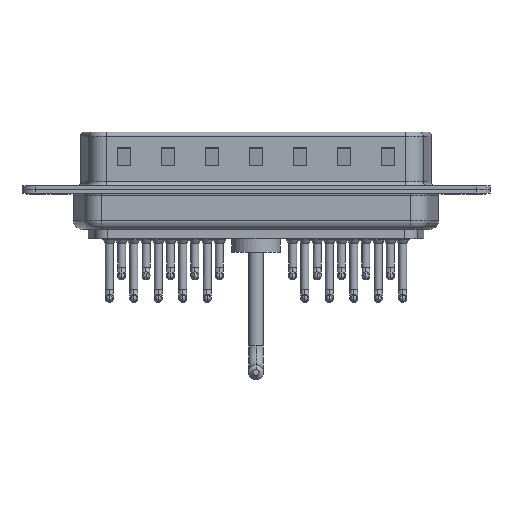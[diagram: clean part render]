
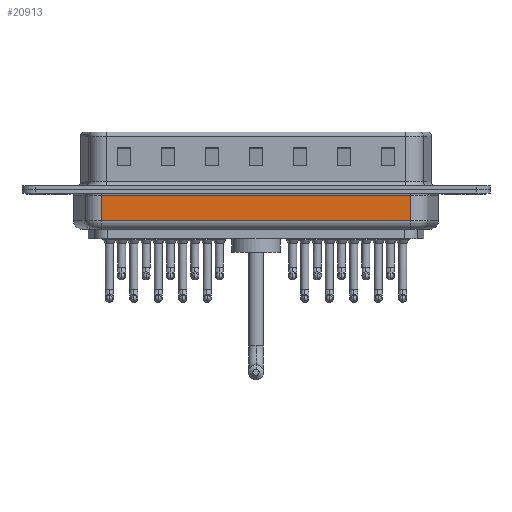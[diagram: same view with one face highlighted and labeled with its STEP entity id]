
A CAD part, front view. The second image highlights one B-rep face of the part: STEP entity #20913.
In plain terms, the highlighted planar face has unit normal (0, -1, 0).
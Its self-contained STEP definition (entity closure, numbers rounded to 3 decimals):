
#125 = CARTESIAN_POINT ( 'NONE',  ( 6.006, -5.35, -0.65 ) ) ;
#293 = ORIENTED_EDGE ( 'NONE', *, *, #11202, .T. ) ;
#4726 = CARTESIAN_POINT ( 'NONE',  ( 6.006, -5.35, -0.65 ) ) ;
#4767 = VECTOR ( 'NONE', #20008, 1000. ) ;
#5064 = FACE_OUTER_BOUND ( 'NONE', #13318, .T. ) ;
#5368 = DIRECTION ( 'NONE',  ( -1., 0., 0. ) ) ;
#5595 = LINE ( 'NONE', #125, #11075 ) ;
#6647 = ORIENTED_EDGE ( 'NONE', *, *, #16174, .T. ) ;
#6909 = VERTEX_POINT ( 'NONE', #4726 ) ;
#7134 = DIRECTION ( 'NONE',  ( 0., 1., 0. ) ) ;
#7353 = LINE ( 'NONE', #11246, #23044 ) ;
#8063 = CARTESIAN_POINT ( 'NONE',  ( 6.006, -5.35, -4.5 ) ) ;
#9010 = CARTESIAN_POINT ( 'NONE',  ( 41.044, -5.35, -3.5 ) ) ;
#9909 = EDGE_CURVE ( 'NONE', #18828, #12997, #12587, .T. ) ;
#10385 = LINE ( 'NONE', #8063, #19255 ) ;
#11061 = CARTESIAN_POINT ( 'NONE',  ( 41.044, -5.35, -0.65 ) ) ;
#11075 = VECTOR ( 'NONE', #5368, 1000. ) ;
#11202 = EDGE_CURVE ( 'NONE', #16367, #6909, #5595, .T. ) ;
#11246 = CARTESIAN_POINT ( 'NONE',  ( 41.044, -5.35, -4.5 ) ) ;
#12587 = LINE ( 'NONE', #21594, #4767 ) ;
#12738 = DIRECTION ( 'NONE',  ( 0., 0., 1. ) ) ;
#12997 = VERTEX_POINT ( 'NONE', #9010 ) ;
#13318 = EDGE_LOOP ( 'NONE', ( #19593, #15335, #6647, #293 ) ) ;
#15335 = ORIENTED_EDGE ( 'NONE', *, *, #9909, .T. ) ;
#16174 = EDGE_CURVE ( 'NONE', #12997, #16367, #7353, .T. ) ;
#16367 = VERTEX_POINT ( 'NONE', #11061 ) ;
#17613 = EDGE_CURVE ( 'NONE', #18828, #6909, #10385, .T. ) ;
#17680 = DIRECTION ( 'NONE',  ( 0., 0., 1. ) ) ;
#18099 = PLANE ( 'NONE',  #20401 ) ;
#18224 = CARTESIAN_POINT ( 'NONE',  ( 6.006, -5.35, -4.5 ) ) ;
#18677 = DIRECTION ( 'NONE',  ( 0., 0., 1. ) ) ;
#18828 = VERTEX_POINT ( 'NONE', #18910 ) ;
#18910 = CARTESIAN_POINT ( 'NONE',  ( 6.006, -5.35, -3.5 ) ) ;
#19255 = VECTOR ( 'NONE', #17680, 1000. ) ;
#19593 = ORIENTED_EDGE ( 'NONE', *, *, #17613, .F. ) ;
#20008 = DIRECTION ( 'NONE',  ( 1., 0., 0. ) ) ;
#20401 = AXIS2_PLACEMENT_3D ( 'NONE', #18224, #7134, #12738 ) ;
#20913 = ADVANCED_FACE ( 'NONE', ( #5064 ), #18099, .F. ) ;
#21594 = CARTESIAN_POINT ( 'NONE',  ( 6.006, -5.35, -3.5 ) ) ;
#23044 = VECTOR ( 'NONE', #18677, 1000. ) ;
